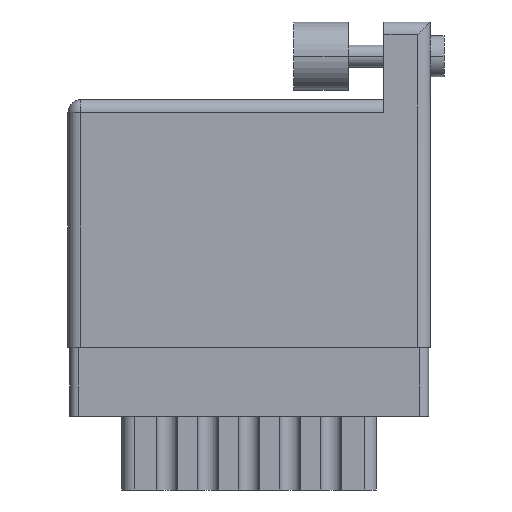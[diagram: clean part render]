
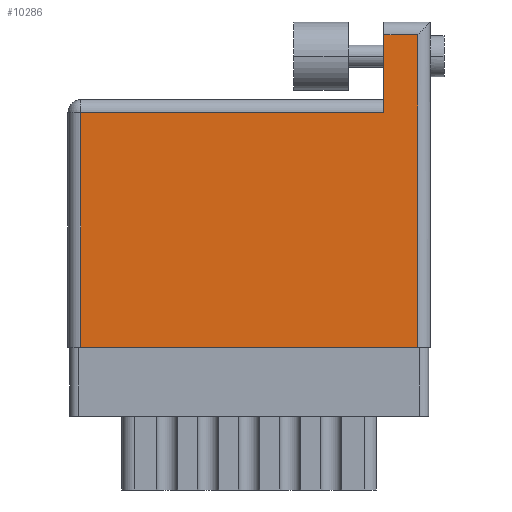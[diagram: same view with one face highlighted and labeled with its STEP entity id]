
A CAD part, front view. The second image highlights one B-rep face of the part: STEP entity #10286.
In plain terms, the highlighted face is planar.
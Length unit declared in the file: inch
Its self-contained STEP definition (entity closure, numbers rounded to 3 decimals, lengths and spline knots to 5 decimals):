
#39 = CARTESIAN_POINT ( 'NONE',  ( 0.047, 0., 0. ) ) ;
#84 = EDGE_LOOP ( 'NONE', ( #9587, #1425, #4598, #8592, #426, #13116 ) ) ;
#142 = PLANE ( 'NONE',  #3822 ) ;
#426 = ORIENTED_EDGE ( 'NONE', *, *, #19672, .T. ) ;
#728 = LINE ( 'NONE', #7301, #5333 ) ;
#1425 = ORIENTED_EDGE ( 'NONE', *, *, #6690, .T. ) ;
#1863 = FACE_OUTER_BOUND ( 'NONE', #84, .T. ) ;
#1976 = LINE ( 'NONE', #39, #9963 ) ;
#2530 = CARTESIAN_POINT ( 'NONE',  ( 1.278, 0., 0. ) ) ;
#2767 = CARTESIAN_POINT ( 'NONE',  ( 0., 0., 0. ) ) ;
#3248 = DIRECTION ( 'NONE',  ( 0., 0., -1. ) ) ;
#3503 = VERTEX_POINT ( 'NONE', #5943 ) ;
#3798 = CARTESIAN_POINT ( 'NONE',  ( 1.155, 1.19, 0. ) ) ;
#3822 = AXIS2_PLACEMENT_3D ( 'NONE', #11705, #3248, #13208 ) ;
#4598 = ORIENTED_EDGE ( 'NONE', *, *, #17698, .T. ) ;
#4749 = EDGE_CURVE ( 'NONE', #10546, #8604, #1976, .T. ) ;
#4935 = VECTOR ( 'NONE', #18682, 39.37008 ) ;
#5333 = VECTOR ( 'NONE', #16906, 39.37008 ) ;
#5943 = CARTESIAN_POINT ( 'NONE',  ( 1.278, 1.143, 0. ) ) ;
#6690 = EDGE_CURVE ( 'NONE', #21181, #3503, #15847, .T. ) ;
#7038 = LINE ( 'NONE', #3798, #4935 ) ;
#7259 = VECTOR ( 'NONE', #20862, 39.37008 ) ;
#7301 = CARTESIAN_POINT ( 'NONE',  ( 1.155, 1.143, 0. ) ) ;
#8592 = ORIENTED_EDGE ( 'NONE', *, *, #15742, .T. ) ;
#8604 = VERTEX_POINT ( 'NONE', #11187 ) ;
#8879 = CARTESIAN_POINT ( 'NONE',  ( 1.155, 0.859, 0. ) ) ;
#9069 = DIRECTION ( 'NONE',  ( -1., 0., 0. ) ) ;
#9587 = ORIENTED_EDGE ( 'NONE', *, *, #13807, .T. ) ;
#9963 = VECTOR ( 'NONE', #14933, 39.37008 ) ;
#10117 = VERTEX_POINT ( 'NONE', #8879 ) ;
#10286 = ADVANCED_FACE ( 'NONE', ( #1863 ), #142, .F. ) ;
#10546 = VERTEX_POINT ( 'NONE', #17479 ) ;
#10599 = CARTESIAN_POINT ( 'NONE',  ( 0., 0.859, 0. ) ) ;
#11187 = CARTESIAN_POINT ( 'NONE',  ( 0.047, 0., 0. ) ) ;
#11705 = CARTESIAN_POINT ( 'NONE',  ( 0., 0.906, 0. ) ) ;
#12738 = VERTEX_POINT ( 'NONE', #20169 ) ;
#12833 = VECTOR ( 'NONE', #20783, 39.37008 ) ;
#13116 = ORIENTED_EDGE ( 'NONE', *, *, #4749, .T. ) ;
#13208 = DIRECTION ( 'NONE',  ( -1., 0., 0. ) ) ;
#13720 = LINE ( 'NONE', #10599, #19825 ) ;
#13807 = EDGE_CURVE ( 'NONE', #8604, #21181, #17544, .T. ) ;
#14254 = CARTESIAN_POINT ( 'NONE',  ( 1.278, 1.19, 0. ) ) ;
#14933 = DIRECTION ( 'NONE',  ( 0., -1., 0. ) ) ;
#15742 = EDGE_CURVE ( 'NONE', #12738, #10117, #7038, .T. ) ;
#15847 = LINE ( 'NONE', #14254, #12833 ) ;
#16906 = DIRECTION ( 'NONE',  ( -1., 0., 0. ) ) ;
#17479 = CARTESIAN_POINT ( 'NONE',  ( 0.047, 0.859, 0. ) ) ;
#17544 = LINE ( 'NONE', #2767, #7259 ) ;
#17698 = EDGE_CURVE ( 'NONE', #3503, #12738, #728, .T. ) ;
#18682 = DIRECTION ( 'NONE',  ( 0., -1., 0. ) ) ;
#19672 = EDGE_CURVE ( 'NONE', #10117, #10546, #13720, .T. ) ;
#19825 = VECTOR ( 'NONE', #9069, 39.37008 ) ;
#20169 = CARTESIAN_POINT ( 'NONE',  ( 1.155, 1.143, 0. ) ) ;
#20783 = DIRECTION ( 'NONE',  ( 0., 1., 0. ) ) ;
#20862 = DIRECTION ( 'NONE',  ( 1., 0., 0. ) ) ;
#21181 = VERTEX_POINT ( 'NONE', #2530 ) ;
